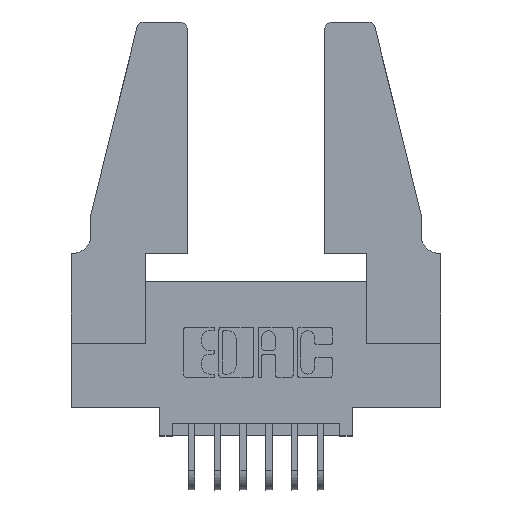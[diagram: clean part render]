
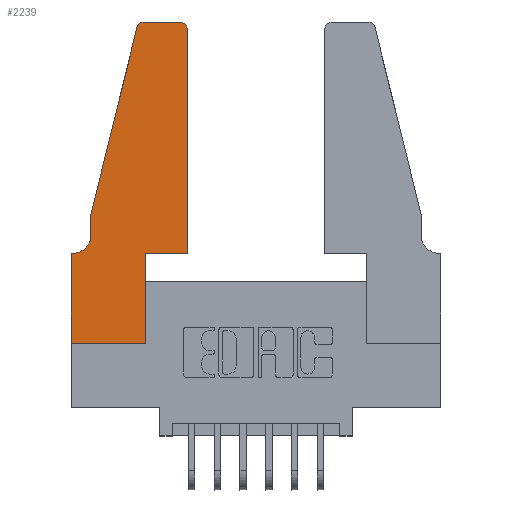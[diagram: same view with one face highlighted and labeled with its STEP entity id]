
A CAD part, top view. The second image highlights one B-rep face of the part: STEP entity #2239.
In plain terms, the highlighted planar face has unit normal (0, 0, 1).
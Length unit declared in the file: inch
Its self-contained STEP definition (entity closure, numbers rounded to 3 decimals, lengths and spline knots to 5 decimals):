
#71 = CIRCLE ( 'NONE', #4731, 0.03 ) ;
#304 = DIRECTION ( 'NONE',  ( 0., 0., 1. ) ) ;
#460 = DIRECTION ( 'NONE',  ( 0., 1., 0. ) ) ;
#498 = LINE ( 'NONE', #11938, #809 ) ;
#511 = VERTEX_POINT ( 'NONE', #8915 ) ;
#642 = VECTOR ( 'NONE', #13005, 39.37008 ) ;
#691 = ORIENTED_EDGE ( 'NONE', *, *, #5922, .T. ) ;
#809 = VECTOR ( 'NONE', #4467, 39.37008 ) ;
#995 = CARTESIAN_POINT ( 'NONE',  ( 0.0755, 0.5, 0.37 ) ) ;
#1016 = CARTESIAN_POINT ( 'NONE',  ( 0.284, 1.22, 0.37 ) ) ;
#1088 = VERTEX_POINT ( 'NONE', #12178 ) ;
#1937 = DIRECTION ( 'NONE',  ( 0., -1., 0. ) ) ;
#2188 = VERTEX_POINT ( 'NONE', #6048 ) ;
#2239 = ADVANCED_FACE ( 'NONE', ( #13346 ), #10729, .T. ) ;
#2403 = DIRECTION ( 'NONE',  ( 1., 0., 0. ) ) ;
#2416 = VECTOR ( 'NONE', #460, 39.37008 ) ;
#2501 = CARTESIAN_POINT ( 'NONE',  ( 0.284, 1.25, 0.37 ) ) ;
#2629 = AXIS2_PLACEMENT_3D ( 'NONE', #1016, #8336, #5183 ) ;
#2894 = CARTESIAN_POINT ( 'NONE',  ( 0., 0., 0.37 ) ) ;
#2907 = CIRCLE ( 'NONE', #2629, 0.03 ) ;
#3521 = CARTESIAN_POINT ( 'NONE',  ( 0.4205, 1.25, 0.37 ) ) ;
#3540 = DIRECTION ( 'NONE',  ( 0., 1., 0. ) ) ;
#3716 = ORIENTED_EDGE ( 'NONE', *, *, #9132, .T. ) ;
#3724 = CARTESIAN_POINT ( 'NONE',  ( 0.2865, 0.35, 0.37 ) ) ;
#3988 = DIRECTION ( 'NONE',  ( 0., -1., 0. ) ) ;
#4050 = ORIENTED_EDGE ( 'NONE', *, *, #8282, .T. ) ;
#4076 = DIRECTION ( 'NONE',  ( 1., 0., 0. ) ) ;
#4114 = ORIENTED_EDGE ( 'NONE', *, *, #7756, .T. ) ;
#4198 = DIRECTION ( 'NONE',  ( -1., 0., 0. ) ) ;
#4371 = LINE ( 'NONE', #995, #8003 ) ;
#4414 = ORIENTED_EDGE ( 'NONE', *, *, #13411, .T. ) ;
#4443 = DIRECTION ( 'NONE',  ( 0., 0., 1. ) ) ;
#4444 = ORIENTED_EDGE ( 'NONE', *, *, #12839, .T. ) ;
#4467 = DIRECTION ( 'NONE',  ( -1., 0., 0. ) ) ;
#4731 = AXIS2_PLACEMENT_3D ( 'NONE', #6594, #304, #2403 ) ;
#4761 = CARTESIAN_POINT ( 'NONE',  ( 0.2605, 1.25, 0.37 ) ) ;
#5000 = ORIENTED_EDGE ( 'NONE', *, *, #8496, .T. ) ;
#5183 = DIRECTION ( 'NONE',  ( 1., 0., 0. ) ) ;
#5189 = LINE ( 'NONE', #4761, #642 ) ;
#5365 = VERTEX_POINT ( 'NONE', #8059 ) ;
#5868 = CARTESIAN_POINT ( 'NONE',  ( 0.0755, 0.42, 0.37 ) ) ;
#5886 = CARTESIAN_POINT ( 'NONE',  ( 0.4505, 0.35, 0.37 ) ) ;
#5922 = EDGE_CURVE ( 'NONE', #11318, #5365, #6462, .T. ) ;
#5926 = VERTEX_POINT ( 'NONE', #5868 ) ;
#6048 = CARTESIAN_POINT ( 'NONE',  ( 0.0055, 0.35, 0.37 ) ) ;
#6144 = ORIENTED_EDGE ( 'NONE', *, *, #7011, .T. ) ;
#6223 = VECTOR ( 'NONE', #3540, 39.37008 ) ;
#6253 = VERTEX_POINT ( 'NONE', #3521 ) ;
#6312 = CARTESIAN_POINT ( 'NONE',  ( 0.25487, 1.22718, 0.37 ) ) ;
#6350 = AXIS2_PLACEMENT_3D ( 'NONE', #8574, #4443, #6425 ) ;
#6425 = DIRECTION ( 'NONE',  ( 1., 0., 0. ) ) ;
#6462 = LINE ( 'NONE', #2894, #10902 ) ;
#6565 = ORIENTED_EDGE ( 'NONE', *, *, #13370, .T. ) ;
#6594 = CARTESIAN_POINT ( 'NONE',  ( 0.4205, 1.22, 0.37 ) ) ;
#6937 = ORIENTED_EDGE ( 'NONE', *, *, #10208, .T. ) ;
#6944 = VECTOR ( 'NONE', #4076, 39.37008 ) ;
#7011 = EDGE_CURVE ( 'NONE', #511, #12154, #11037, .T. ) ;
#7228 = LINE ( 'NONE', #12930, #6223 ) ;
#7308 = CARTESIAN_POINT ( 'NONE',  ( 0., 0., 0.37 ) ) ;
#7756 = EDGE_CURVE ( 'NONE', #11638, #5926, #11338, .T. ) ;
#8003 = VECTOR ( 'NONE', #9360, 39.37008 ) ;
#8041 = VECTOR ( 'NONE', #3988, 39.37008 ) ;
#8059 = CARTESIAN_POINT ( 'NONE',  ( 0.2865, 0., 0.37 ) ) ;
#8282 = EDGE_CURVE ( 'NONE', #12154, #10228, #7228, .T. ) ;
#8305 = CIRCLE ( 'NONE', #10025, 0.07 ) ;
#8336 = DIRECTION ( 'NONE',  ( 0., 0., 1. ) ) ;
#8363 = CARTESIAN_POINT ( 'NONE',  ( 0.0055, 0.42, 0.37 ) ) ;
#8369 = VECTOR ( 'NONE', #1937, 39.37008 ) ;
#8496 = EDGE_CURVE ( 'NONE', #1088, #11318, #10649, .T. ) ;
#8574 = CARTESIAN_POINT ( 'NONE',  ( 0., 0.35, 0.37 ) ) ;
#8582 = EDGE_LOOP ( 'NONE', ( #10129, #9611, #6565, #4114, #4414, #3716, #5000, #691, #4444, #6144, #4050, #6937 ) ) ;
#8915 = CARTESIAN_POINT ( 'NONE',  ( 0.2865, 0.35, 0.37 ) ) ;
#8973 = LINE ( 'NONE', #3724, #2416 ) ;
#9121 = VERTEX_POINT ( 'NONE', #2501 ) ;
#9132 = EDGE_CURVE ( 'NONE', #2188, #1088, #498, .T. ) ;
#9360 = DIRECTION ( 'NONE',  ( -0.239, -0.971, 0. ) ) ;
#9410 = DIRECTION ( 'NONE',  ( 0., 0., -1. ) ) ;
#9611 = ORIENTED_EDGE ( 'NONE', *, *, #9654, .T. ) ;
#9654 = EDGE_CURVE ( 'NONE', #9121, #12523, #2907, .T. ) ;
#9936 = EDGE_CURVE ( 'NONE', #6253, #9121, #5189, .T. ) ;
#10025 = AXIS2_PLACEMENT_3D ( 'NONE', #8363, #9410, #4198 ) ;
#10091 = DIRECTION ( 'NONE',  ( 1., 0., 0. ) ) ;
#10129 = ORIENTED_EDGE ( 'NONE', *, *, #9936, .T. ) ;
#10208 = EDGE_CURVE ( 'NONE', #10228, #6253, #71, .T. ) ;
#10228 = VERTEX_POINT ( 'NONE', #12626 ) ;
#10349 = CARTESIAN_POINT ( 'NONE',  ( 0.4505, 0.35, 0.37 ) ) ;
#10649 = LINE ( 'NONE', #7308, #8041 ) ;
#10729 = PLANE ( 'NONE',  #6350 ) ;
#10902 = VECTOR ( 'NONE', #10091, 39.37008 ) ;
#11037 = LINE ( 'NONE', #10349, #6944 ) ;
#11318 = VERTEX_POINT ( 'NONE', #12788 ) ;
#11338 = LINE ( 'NONE', #13434, #8369 ) ;
#11638 = VERTEX_POINT ( 'NONE', #12139 ) ;
#11938 = CARTESIAN_POINT ( 'NONE',  ( 0.0755, 0.35, 0.37 ) ) ;
#12139 = CARTESIAN_POINT ( 'NONE',  ( 0.0755, 0.5, 0.37 ) ) ;
#12154 = VERTEX_POINT ( 'NONE', #5886 ) ;
#12178 = CARTESIAN_POINT ( 'NONE',  ( 0., 0.35, 0.37 ) ) ;
#12523 = VERTEX_POINT ( 'NONE', #6312 ) ;
#12626 = CARTESIAN_POINT ( 'NONE',  ( 0.4505, 1.22, 0.37 ) ) ;
#12788 = CARTESIAN_POINT ( 'NONE',  ( 0., 0., 0.37 ) ) ;
#12839 = EDGE_CURVE ( 'NONE', #5365, #511, #8973, .T. ) ;
#12930 = CARTESIAN_POINT ( 'NONE',  ( 0.4505, 0.35, 0.37 ) ) ;
#13005 = DIRECTION ( 'NONE',  ( -1., 0., 0. ) ) ;
#13346 = FACE_OUTER_BOUND ( 'NONE', #8582, .T. ) ;
#13370 = EDGE_CURVE ( 'NONE', #12523, #11638, #4371, .T. ) ;
#13411 = EDGE_CURVE ( 'NONE', #5926, #2188, #8305, .T. ) ;
#13434 = CARTESIAN_POINT ( 'NONE',  ( 0.0755, 0.5, 0.37 ) ) ;
